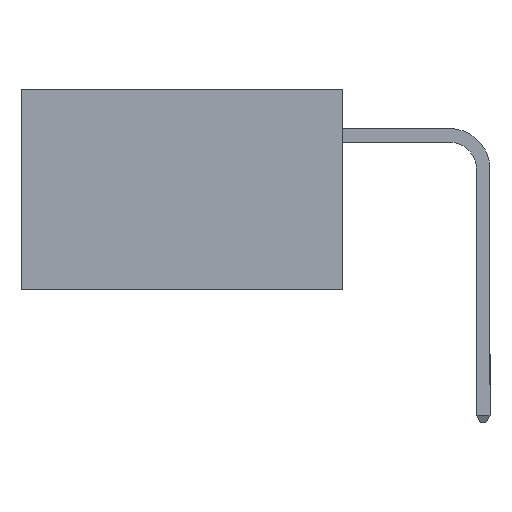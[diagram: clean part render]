
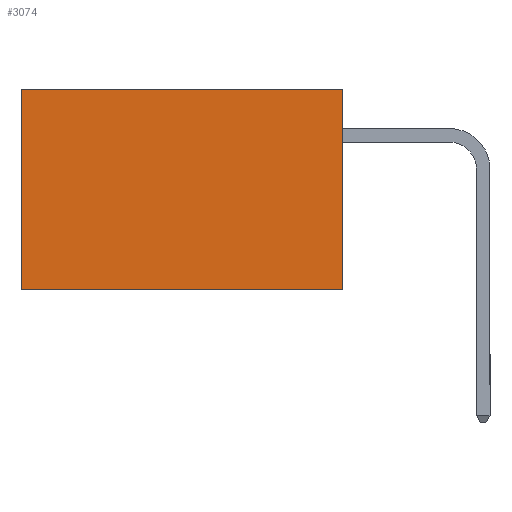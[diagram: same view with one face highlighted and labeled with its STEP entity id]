
A CAD part, left-side view. The second image highlights one B-rep face of the part: STEP entity #3074.
In plain terms, the highlighted planar face has unit normal (-1, 0, 0).
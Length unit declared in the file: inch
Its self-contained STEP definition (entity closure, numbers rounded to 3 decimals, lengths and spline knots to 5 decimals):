
#49 = DIRECTION ( 'NONE',  ( 0., 1., 0. ) ) ;
#672 = VECTOR ( 'NONE', #2291, 39.37008 ) ;
#1021 = LINE ( 'NONE', #1222, #672 ) ;
#1219 = VECTOR ( 'NONE', #8292, 39.37008 ) ;
#1222 = CARTESIAN_POINT ( 'NONE',  ( 0.277, 0., -0.37 ) ) ;
#1351 = CARTESIAN_POINT ( 'NONE',  ( 0.277, 0.59, -0.37 ) ) ;
#1374 = VECTOR ( 'NONE', #8291, 39.37008 ) ;
#1481 = EDGE_CURVE ( 'NONE', #5978, #7823, #10931, .T. ) ;
#2097 = EDGE_CURVE ( 'NONE', #5978, #11857, #6453, .T. ) ;
#2230 = CARTESIAN_POINT ( 'NONE',  ( 0.277, 0., -0.37 ) ) ;
#2291 = DIRECTION ( 'NONE',  ( 0., 1., 0. ) ) ;
#2675 = EDGE_LOOP ( 'NONE', ( #11816, #8744, #8796, #8680 ) ) ;
#2689 = CARTESIAN_POINT ( 'NONE',  ( 0.277, 0., 0. ) ) ;
#3074 = ADVANCED_FACE ( 'NONE', ( #13272 ), #9179, .F. ) ;
#4933 = VERTEX_POINT ( 'NONE', #1351 ) ;
#5978 = VERTEX_POINT ( 'NONE', #2689 ) ;
#6453 = LINE ( 'NONE', #8411, #1374 ) ;
#6639 = CARTESIAN_POINT ( 'NONE',  ( 0.277, 0.59, 0. ) ) ;
#7823 = VERTEX_POINT ( 'NONE', #6639 ) ;
#8002 = CARTESIAN_POINT ( 'NONE',  ( 0.277, 0., -0.37 ) ) ;
#8207 = AXIS2_PLACEMENT_3D ( 'NONE', #8002, #9205, #9181 ) ;
#8291 = DIRECTION ( 'NONE',  ( 0., 0., -1. ) ) ;
#8292 = DIRECTION ( 'NONE',  ( 0., 0., -1. ) ) ;
#8411 = CARTESIAN_POINT ( 'NONE',  ( 0.277, 0., -0.37 ) ) ;
#8680 = ORIENTED_EDGE ( 'NONE', *, *, #1481, .T. ) ;
#8744 = ORIENTED_EDGE ( 'NONE', *, *, #12995, .F. ) ;
#8796 = ORIENTED_EDGE ( 'NONE', *, *, #2097, .F. ) ;
#9179 = PLANE ( 'NONE',  #8207 ) ;
#9181 = DIRECTION ( 'NONE',  ( 0., 0., -1. ) ) ;
#9205 = DIRECTION ( 'NONE',  ( 1., 0., 0. ) ) ;
#10628 = VECTOR ( 'NONE', #49, 39.37008 ) ;
#10931 = LINE ( 'NONE', #11921, #10628 ) ;
#11816 = ORIENTED_EDGE ( 'NONE', *, *, #12808, .T. ) ;
#11820 = LINE ( 'NONE', #13071, #1219 ) ;
#11857 = VERTEX_POINT ( 'NONE', #2230 ) ;
#11921 = CARTESIAN_POINT ( 'NONE',  ( 0.277, 0., 0. ) ) ;
#12808 = EDGE_CURVE ( 'NONE', #7823, #4933, #11820, .T. ) ;
#12995 = EDGE_CURVE ( 'NONE', #11857, #4933, #1021, .T. ) ;
#13071 = CARTESIAN_POINT ( 'NONE',  ( 0.277, 0.59, -0.37 ) ) ;
#13272 = FACE_OUTER_BOUND ( 'NONE', #2675, .T. ) ;
